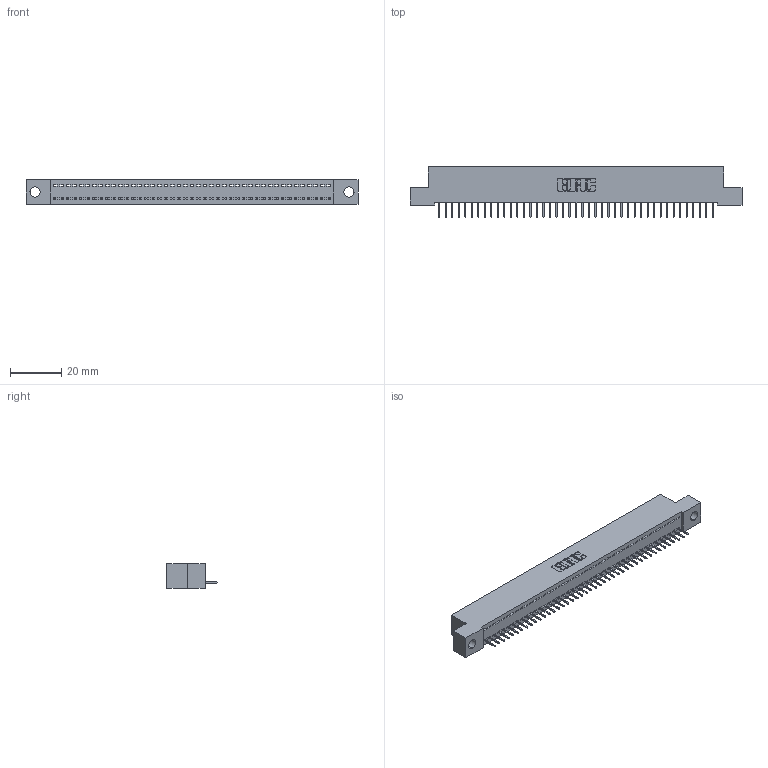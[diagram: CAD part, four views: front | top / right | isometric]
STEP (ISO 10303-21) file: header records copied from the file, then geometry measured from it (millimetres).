
FILE_DESCRIPTION (( 'STEP AP203' ), '1' );
FILE_NAME ('392-043-524-104.STEP', '2018-08-16T14:21:04', ( '' ), ( '' ), 'SwSTEP 2.0', 'SolidWorks 2016', '' );
FILE_SCHEMA (( 'CONFIG_CONTROL_DESIGN' ));
Length unit declared in the file: inch
Products named in the file (3): 392-043-524-104; 342 Part_.156 TH; 345-292-001_345-293-124
Assembly tree (44 placements, depth 2):
  392-043-524-104
    342 Part_.156 TH
    345-292-001_345-293-124  x43
Bounding box: 129.54 x 19.69 x 9.4 mm (x, y, z)
Volume: 11104.9 mm3; surface area: 15616.8 mm2
Topology: 44 solids, 44 shells, 2776 faces, 8039 edges, 5186 vertices
Faces by surface type: plane 2130, cylinder 646
Entity records: 26103 total; most frequent: CARTESIAN_POINT 4507, ORIENTED_EDGE 4486, DIRECTION 3801, EDGE_CURVE 2243, LINE 2119, VECTOR 2119, VERTEX_POINT 1490, AXIS2_PLACEMENT_3D 841
